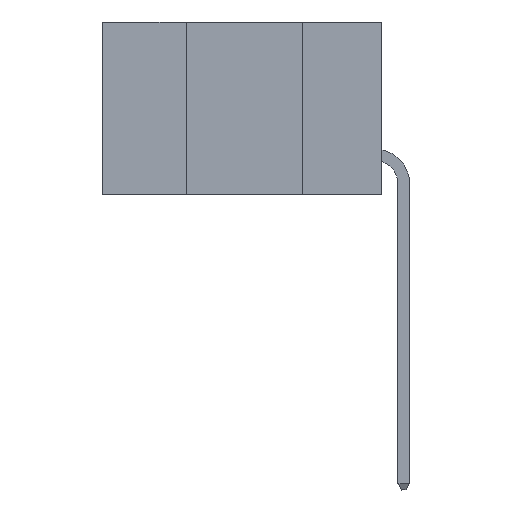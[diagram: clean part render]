
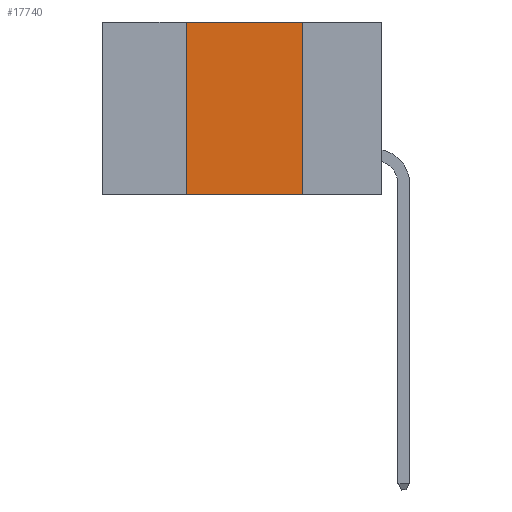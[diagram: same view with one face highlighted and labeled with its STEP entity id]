
A CAD part, left-side view. The second image highlights one B-rep face of the part: STEP entity #17740.
In plain terms, the highlighted planar face has unit normal (-1, 0, 0).
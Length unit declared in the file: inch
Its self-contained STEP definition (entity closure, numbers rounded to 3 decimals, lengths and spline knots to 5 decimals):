
#109 = AXIS2_PLACEMENT_3D ( 'NONE', #14810, #2495, #12844 ) ;
#660 = DIRECTION ( 'NONE',  ( 0., -1., 0. ) ) ;
#1007 = LINE ( 'NONE', #15336, #17852 ) ;
#1530 = CARTESIAN_POINT ( 'NONE',  ( 0., 0.17, 0. ) ) ;
#2476 = ORIENTED_EDGE ( 'NONE', *, *, #14573, .F. ) ;
#2495 = DIRECTION ( 'NONE',  ( 1., 0., 0. ) ) ;
#2833 = CARTESIAN_POINT ( 'NONE',  ( 0., 0.42, -0.37 ) ) ;
#3235 = DIRECTION ( 'NONE',  ( 0., 0., -1. ) ) ;
#4230 = VERTEX_POINT ( 'NONE', #2833 ) ;
#4529 = LINE ( 'NONE', #1530, #9695 ) ;
#6045 = PLANE ( 'NONE',  #109 ) ;
#6311 = ORIENTED_EDGE ( 'NONE', *, *, #8458, .F. ) ;
#7159 = FACE_OUTER_BOUND ( 'NONE', #13735, .T. ) ;
#8458 = EDGE_CURVE ( 'NONE', #10172, #9371, #20945, .T. ) ;
#9248 = VECTOR ( 'NONE', #21814, 39.37008 ) ;
#9371 = VERTEX_POINT ( 'NONE', #17897 ) ;
#9695 = VECTOR ( 'NONE', #3235, 39.37008 ) ;
#9739 = CARTESIAN_POINT ( 'NONE',  ( 0., 0.42, 0. ) ) ;
#10172 = VERTEX_POINT ( 'NONE', #16733 ) ;
#10967 = DIRECTION ( 'NONE',  ( 0., -1., 0. ) ) ;
#11179 = VECTOR ( 'NONE', #10967, 39.37008 ) ;
#12751 = ORIENTED_EDGE ( 'NONE', *, *, #21213, .F. ) ;
#12844 = DIRECTION ( 'NONE',  ( 0., 0., -1. ) ) ;
#13735 = EDGE_LOOP ( 'NONE', ( #12751, #6311, #2476, #14173 ) ) ;
#14173 = ORIENTED_EDGE ( 'NONE', *, *, #19775, .T. ) ;
#14573 = EDGE_CURVE ( 'NONE', #4230, #10172, #15784, .T. ) ;
#14810 = CARTESIAN_POINT ( 'NONE',  ( 0., 0.6, 0. ) ) ;
#15336 = CARTESIAN_POINT ( 'NONE',  ( 0., 0.6, -0.37 ) ) ;
#15784 = LINE ( 'NONE', #9739, #9248 ) ;
#16733 = CARTESIAN_POINT ( 'NONE',  ( 0., 0.42, 0. ) ) ;
#17285 = CARTESIAN_POINT ( 'NONE',  ( 0., 0.17, -0.37 ) ) ;
#17740 = ADVANCED_FACE ( 'NONE', ( #7159 ), #6045, .F. ) ;
#17844 = CARTESIAN_POINT ( 'NONE',  ( 0., 0.6, 0. ) ) ;
#17852 = VECTOR ( 'NONE', #660, 39.37008 ) ;
#17897 = CARTESIAN_POINT ( 'NONE',  ( 0., 0.17, 0. ) ) ;
#19775 = EDGE_CURVE ( 'NONE', #4230, #22054, #1007, .T. ) ;
#20945 = LINE ( 'NONE', #17844, #11179 ) ;
#21213 = EDGE_CURVE ( 'NONE', #9371, #22054, #4529, .T. ) ;
#21814 = DIRECTION ( 'NONE',  ( 0., 0., 1. ) ) ;
#22054 = VERTEX_POINT ( 'NONE', #17285 ) ;
